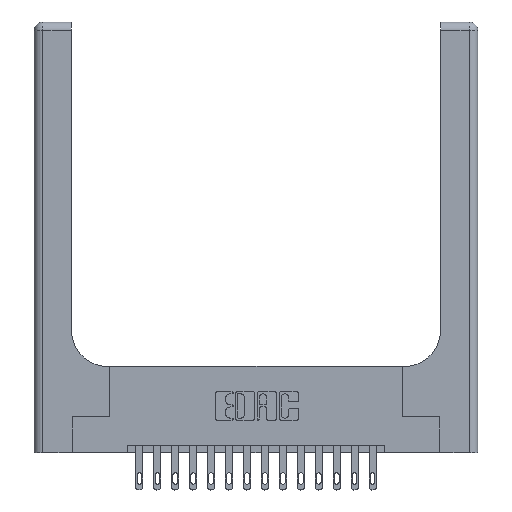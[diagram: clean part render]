
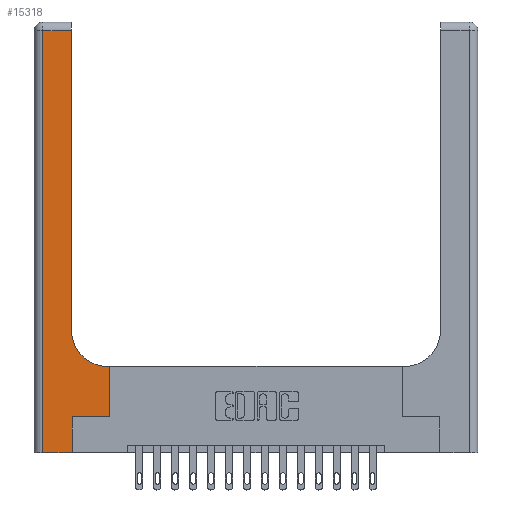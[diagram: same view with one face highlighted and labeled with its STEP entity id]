
A CAD part, top view. The second image highlights one B-rep face of the part: STEP entity #15318.
In plain terms, the highlighted planar face has unit normal (0, 0, 1).
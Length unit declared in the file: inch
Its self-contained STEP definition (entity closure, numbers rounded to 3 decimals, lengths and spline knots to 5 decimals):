
#373 = CIRCLE ( 'NONE', #13218, 0.25 ) ;
#527 = VECTOR ( 'NONE', #16522, 39.37008 ) ;
#539 = LINE ( 'NONE', #10616, #12765 ) ;
#571 = DIRECTION ( 'NONE',  ( 0., -1., 0. ) ) ;
#573 = DIRECTION ( 'NONE',  ( 1., 0., 0. ) ) ;
#837 = LINE ( 'NONE', #4958, #527 ) ;
#1091 = PLANE ( 'NONE',  #9399 ) ;
#1591 = CARTESIAN_POINT ( 'NONE',  ( 0.26, 2.94, 0.37 ) ) ;
#1699 = EDGE_LOOP ( 'NONE', ( #12957, #9382, #6118, #3453, #18059, #3496, #2581, #5201, #16514 ) ) ;
#1908 = CARTESIAN_POINT ( 'NONE',  ( 0.26, 0.85, 0.37 ) ) ;
#2075 = LINE ( 'NONE', #14910, #13759 ) ;
#2078 = DIRECTION ( 'NONE',  ( 1., 0., 0. ) ) ;
#2363 = VERTEX_POINT ( 'NONE', #2634 ) ;
#2402 = VERTEX_POINT ( 'NONE', #17448 ) ;
#2581 = ORIENTED_EDGE ( 'NONE', *, *, #3580, .T. ) ;
#2634 = CARTESIAN_POINT ( 'NONE',  ( 0.265, 0.25, 0.37 ) ) ;
#3453 = ORIENTED_EDGE ( 'NONE', *, *, #4679, .T. ) ;
#3496 = ORIENTED_EDGE ( 'NONE', *, *, #7062, .T. ) ;
#3580 = EDGE_CURVE ( 'NONE', #11794, #15462, #8430, .T. ) ;
#3627 = VECTOR ( 'NONE', #11005, 39.37008 ) ;
#3805 = VERTEX_POINT ( 'NONE', #1591 ) ;
#4584 = VECTOR ( 'NONE', #2078, 39.37008 ) ;
#4679 = EDGE_CURVE ( 'NONE', #2402, #5833, #15633, .T. ) ;
#4958 = CARTESIAN_POINT ( 'NONE',  ( 0.26, 3., 0.37 ) ) ;
#5201 = ORIENTED_EDGE ( 'NONE', *, *, #8655, .T. ) ;
#5360 = VERTEX_POINT ( 'NONE', #17753 ) ;
#5364 = EDGE_CURVE ( 'NONE', #9119, #10607, #373, .T. ) ;
#5391 = FACE_OUTER_BOUND ( 'NONE', #1699, .T. ) ;
#5833 = VERTEX_POINT ( 'NONE', #13318 ) ;
#6118 = ORIENTED_EDGE ( 'NONE', *, *, #13110, .T. ) ;
#6248 = DIRECTION ( 'NONE',  ( -1., 0., 0. ) ) ;
#6895 = DIRECTION ( 'NONE',  ( -1., 0., 0. ) ) ;
#6921 = LINE ( 'NONE', #8221, #9082 ) ;
#7062 = EDGE_CURVE ( 'NONE', #2363, #11794, #6921, .T. ) ;
#7085 = EDGE_CURVE ( 'NONE', #3805, #5360, #8315, .T. ) ;
#8025 = DIRECTION ( 'NONE',  ( 1., 0., 0. ) ) ;
#8209 = VECTOR ( 'NONE', #9617, 39.37008 ) ;
#8221 = CARTESIAN_POINT ( 'NONE',  ( 0.265, 0.25, 0.37 ) ) ;
#8315 = LINE ( 'NONE', #15374, #8209 ) ;
#8430 = LINE ( 'NONE', #14096, #3627 ) ;
#8640 = CARTESIAN_POINT ( 'NONE',  ( 0.528, 0.6, 0.37 ) ) ;
#8647 = LINE ( 'NONE', #14319, #11307 ) ;
#8655 = EDGE_CURVE ( 'NONE', #15462, #9119, #539, .T. ) ;
#8939 = EDGE_CURVE ( 'NONE', #5833, #2363, #8647, .T. ) ;
#9082 = VECTOR ( 'NONE', #8025, 39.37008 ) ;
#9119 = VERTEX_POINT ( 'NONE', #11432 ) ;
#9382 = ORIENTED_EDGE ( 'NONE', *, *, #7085, .T. ) ;
#9399 = AXIS2_PLACEMENT_3D ( 'NONE', #12368, #15053, #6895 ) ;
#9617 = DIRECTION ( 'NONE',  ( -1., 0., 0. ) ) ;
#10067 = CARTESIAN_POINT ( 'NONE',  ( 0.528, 0.25, 0.37 ) ) ;
#10607 = VERTEX_POINT ( 'NONE', #1908 ) ;
#10616 = CARTESIAN_POINT ( 'NONE',  ( 0.26, 0.6, 0.37 ) ) ;
#10650 = CARTESIAN_POINT ( 'NONE',  ( 0., 0., 0.37 ) ) ;
#11005 = DIRECTION ( 'NONE',  ( 0., 1., 0. ) ) ;
#11079 = EDGE_CURVE ( 'NONE', #10607, #3805, #837, .T. ) ;
#11307 = VECTOR ( 'NONE', #11344, 39.37008 ) ;
#11344 = DIRECTION ( 'NONE',  ( 0., 1., 0. ) ) ;
#11432 = CARTESIAN_POINT ( 'NONE',  ( 0.51, 0.6, 0.37 ) ) ;
#11794 = VERTEX_POINT ( 'NONE', #10067 ) ;
#12368 = CARTESIAN_POINT ( 'NONE',  ( 0., 3., 0.37 ) ) ;
#12765 = VECTOR ( 'NONE', #6248, 39.37008 ) ;
#12957 = ORIENTED_EDGE ( 'NONE', *, *, #11079, .T. ) ;
#13110 = EDGE_CURVE ( 'NONE', #5360, #2402, #2075, .T. ) ;
#13218 = AXIS2_PLACEMENT_3D ( 'NONE', #13339, #17660, #573 ) ;
#13318 = CARTESIAN_POINT ( 'NONE',  ( 0.265, 0., 0.37 ) ) ;
#13339 = CARTESIAN_POINT ( 'NONE',  ( 0.51, 0.85, 0.37 ) ) ;
#13759 = VECTOR ( 'NONE', #571, 39.37008 ) ;
#14096 = CARTESIAN_POINT ( 'NONE',  ( 0.528, 0.25, 0.37 ) ) ;
#14319 = CARTESIAN_POINT ( 'NONE',  ( 0.265, 0., 0.37 ) ) ;
#14910 = CARTESIAN_POINT ( 'NONE',  ( 0.06, 3., 0.37 ) ) ;
#15053 = DIRECTION ( 'NONE',  ( 0., 0., -1. ) ) ;
#15318 = ADVANCED_FACE ( 'NONE', ( #5391 ), #1091, .F. ) ;
#15374 = CARTESIAN_POINT ( 'NONE',  ( 0., 2.94, 0.37 ) ) ;
#15462 = VERTEX_POINT ( 'NONE', #8640 ) ;
#15633 = LINE ( 'NONE', #10650, #4584 ) ;
#16514 = ORIENTED_EDGE ( 'NONE', *, *, #5364, .T. ) ;
#16522 = DIRECTION ( 'NONE',  ( 0., 1., 0. ) ) ;
#17448 = CARTESIAN_POINT ( 'NONE',  ( 0.06, 0., 0.37 ) ) ;
#17660 = DIRECTION ( 'NONE',  ( 0., 0., -1. ) ) ;
#17753 = CARTESIAN_POINT ( 'NONE',  ( 0.06, 2.94, 0.37 ) ) ;
#18059 = ORIENTED_EDGE ( 'NONE', *, *, #8939, .T. ) ;
